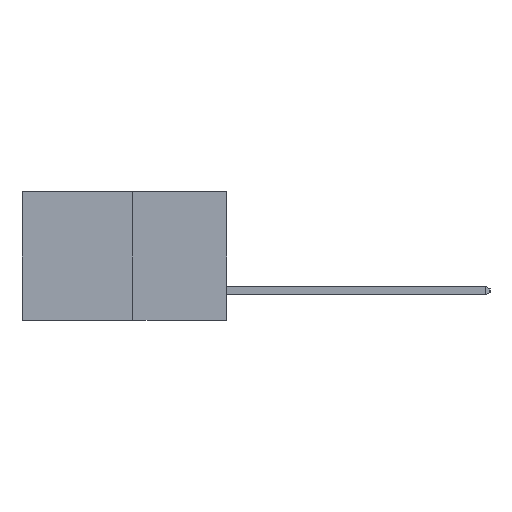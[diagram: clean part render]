
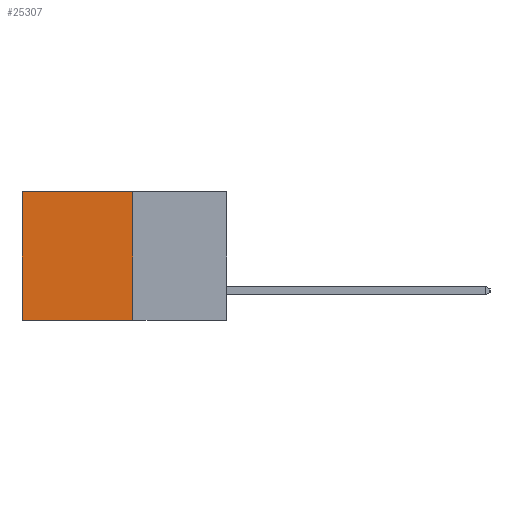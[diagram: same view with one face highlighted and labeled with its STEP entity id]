
A CAD part, left-side view. The second image highlights one B-rep face of the part: STEP entity #25307.
In plain terms, the highlighted planar face has unit normal (-1, 0, 0).
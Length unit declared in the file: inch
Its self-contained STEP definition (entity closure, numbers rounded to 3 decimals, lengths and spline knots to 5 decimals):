
#1140 = EDGE_CURVE ( 'NONE', #19415, #18036, #22822, .T. ) ;
#1880 = CARTESIAN_POINT ( 'NONE',  ( 0.277, 0.59, -0.37 ) ) ;
#2131 = VECTOR ( 'NONE', #8817, 39.37008 ) ;
#2704 = VERTEX_POINT ( 'NONE', #16546 ) ;
#2922 = EDGE_CURVE ( 'NONE', #2704, #18036, #5022, .T. ) ;
#3957 = DIRECTION ( 'NONE',  ( 0., 0., -1. ) ) ;
#4374 = PLANE ( 'NONE',  #7587 ) ;
#4764 = VECTOR ( 'NONE', #3957, 39.37008 ) ;
#5022 = LINE ( 'NONE', #10480, #25431 ) ;
#5712 = ORIENTED_EDGE ( 'NONE', *, *, #2922, .F. ) ;
#6339 = DIRECTION ( 'NONE',  ( 1., 0., 0. ) ) ;
#7587 = AXIS2_PLACEMENT_3D ( 'NONE', #24145, #6339, #20312 ) ;
#8817 = DIRECTION ( 'NONE',  ( 0., 0., -1. ) ) ;
#9637 = DIRECTION ( 'NONE',  ( 0., 1., 0. ) ) ;
#9923 = ORIENTED_EDGE ( 'NONE', *, *, #1140, .T. ) ;
#10480 = CARTESIAN_POINT ( 'NONE',  ( 0.277, 0.27, -0.37 ) ) ;
#10626 = VECTOR ( 'NONE', #25070, 39.37008 ) ;
#11252 = LINE ( 'NONE', #21192, #10626 ) ;
#11483 = CARTESIAN_POINT ( 'NONE',  ( 0.277, 0.27, 0. ) ) ;
#12762 = LINE ( 'NONE', #22772, #2131 ) ;
#13415 = EDGE_LOOP ( 'NONE', ( #9923, #5712, #22830, #20974 ) ) ;
#13856 = VERTEX_POINT ( 'NONE', #11483 ) ;
#13923 = FACE_OUTER_BOUND ( 'NONE', #13415, .T. ) ;
#14269 = CARTESIAN_POINT ( 'NONE',  ( 0.277, 0.59, -0.37 ) ) ;
#16308 = EDGE_CURVE ( 'NONE', #13856, #2704, #12762, .T. ) ;
#16546 = CARTESIAN_POINT ( 'NONE',  ( 0.277, 0.27, -0.37 ) ) ;
#18036 = VERTEX_POINT ( 'NONE', #14269 ) ;
#19415 = VERTEX_POINT ( 'NONE', #20204 ) ;
#20204 = CARTESIAN_POINT ( 'NONE',  ( 0.277, 0.59, 0. ) ) ;
#20312 = DIRECTION ( 'NONE',  ( 0., 0., -1. ) ) ;
#20974 = ORIENTED_EDGE ( 'NONE', *, *, #23183, .T. ) ;
#21192 = CARTESIAN_POINT ( 'NONE',  ( 0.277, 0.27, 0. ) ) ;
#22772 = CARTESIAN_POINT ( 'NONE',  ( 0.277, 0.27, -0.37 ) ) ;
#22822 = LINE ( 'NONE', #1880, #4764 ) ;
#22830 = ORIENTED_EDGE ( 'NONE', *, *, #16308, .F. ) ;
#23183 = EDGE_CURVE ( 'NONE', #13856, #19415, #11252, .T. ) ;
#24145 = CARTESIAN_POINT ( 'NONE',  ( 0.277, 0.27, -0.37 ) ) ;
#25070 = DIRECTION ( 'NONE',  ( 0., 1., 0. ) ) ;
#25307 = ADVANCED_FACE ( 'NONE', ( #13923 ), #4374, .F. ) ;
#25431 = VECTOR ( 'NONE', #9637, 39.37008 ) ;
